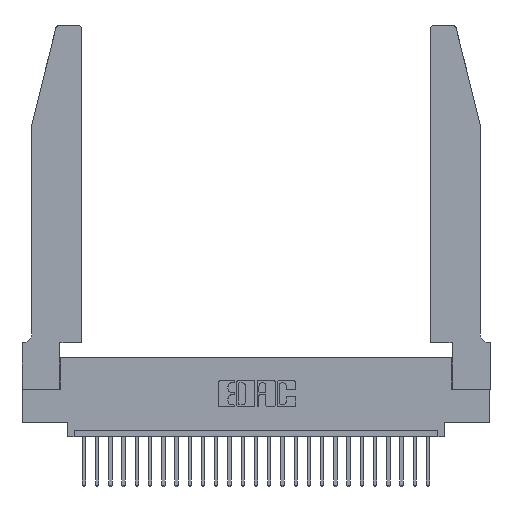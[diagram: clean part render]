
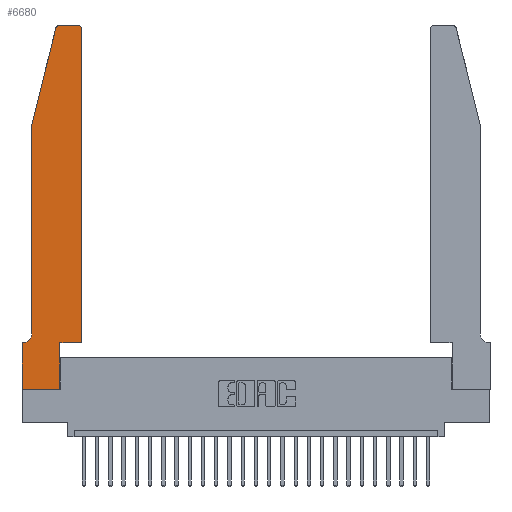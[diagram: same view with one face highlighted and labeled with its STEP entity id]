
A CAD part, top view. The second image highlights one B-rep face of the part: STEP entity #6680.
In plain terms, the highlighted planar face has unit normal (0, 0, 1).
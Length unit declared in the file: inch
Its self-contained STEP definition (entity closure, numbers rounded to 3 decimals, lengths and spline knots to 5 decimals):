
#149 = AXIS2_PLACEMENT_3D ( 'NONE', #14647, #1653, #1747 ) ;
#470 = ORIENTED_EDGE ( 'NONE', *, *, #9379, .T. ) ;
#734 = CIRCLE ( 'NONE', #1820, 0.03 ) ;
#816 = LINE ( 'NONE', #3206, #12697 ) ;
#826 = EDGE_CURVE ( 'NONE', #24561, #16037, #7368, .T. ) ;
#1127 = CARTESIAN_POINT ( 'NONE',  ( 0.2865, 0.35, 0.37 ) ) ;
#1187 = DIRECTION ( 'NONE',  ( 0., -1., 0. ) ) ;
#1245 = CIRCLE ( 'NONE', #149, 0.03 ) ;
#1454 = VERTEX_POINT ( 'NONE', #12712 ) ;
#1579 = CARTESIAN_POINT ( 'NONE',  ( 0.4505, 0.35, 0.37 ) ) ;
#1596 = CARTESIAN_POINT ( 'NONE',  ( 0., 0., 0.37 ) ) ;
#1653 = DIRECTION ( 'NONE',  ( 0., 0., 1. ) ) ;
#1747 = DIRECTION ( 'NONE',  ( 1., 0., 0. ) ) ;
#1820 = AXIS2_PLACEMENT_3D ( 'NONE', #4188, #27153, #19090 ) ;
#1962 = VECTOR ( 'NONE', #13848, 39.37008 ) ;
#3035 = DIRECTION ( 'NONE',  ( -1., 0., 0. ) ) ;
#3103 = EDGE_LOOP ( 'NONE', ( #20905, #11108, #470, #25592, #26043, #8160, #9879, #19861, #3679, #4403, #20275, #17504 ) ) ;
#3206 = CARTESIAN_POINT ( 'NONE',  ( 0.4505, 0.35, 0.37 ) ) ;
#3237 = VERTEX_POINT ( 'NONE', #6074 ) ;
#3348 = CARTESIAN_POINT ( 'NONE',  ( 0., 0., 0.37 ) ) ;
#3528 = VERTEX_POINT ( 'NONE', #17537 ) ;
#3679 = ORIENTED_EDGE ( 'NONE', *, *, #6394, .T. ) ;
#4188 = CARTESIAN_POINT ( 'NONE',  ( 0.4205, 2.72, 0.37 ) ) ;
#4379 = CARTESIAN_POINT ( 'NONE',  ( 0.4505, 2.72, 0.37 ) ) ;
#4403 = ORIENTED_EDGE ( 'NONE', *, *, #11843, .T. ) ;
#6074 = CARTESIAN_POINT ( 'NONE',  ( 0.25487, 2.72718, 0.37 ) ) ;
#6394 = EDGE_CURVE ( 'NONE', #25896, #17495, #16190, .T. ) ;
#6680 = ADVANCED_FACE ( 'NONE', ( #23380 ), #14019, .T. ) ;
#7368 = LINE ( 'NONE', #23674, #12301 ) ;
#8012 = CARTESIAN_POINT ( 'NONE',  ( 0., 0.35, 0.37 ) ) ;
#8160 = ORIENTED_EDGE ( 'NONE', *, *, #826, .T. ) ;
#8242 = CARTESIAN_POINT ( 'NONE',  ( 0.2605, 2.75, 0.37 ) ) ;
#8655 = CARTESIAN_POINT ( 'NONE',  ( 0.2865, 0.35, 0.37 ) ) ;
#8713 = LINE ( 'NONE', #3348, #20563 ) ;
#8955 = EDGE_CURVE ( 'NONE', #20782, #3528, #13169, .T. ) ;
#9379 = EDGE_CURVE ( 'NONE', #3237, #26907, #14814, .T. ) ;
#9433 = EDGE_CURVE ( 'NONE', #27029, #25896, #15794, .T. ) ;
#9781 = CARTESIAN_POINT ( 'NONE',  ( 0.0755, 2., 0.37 ) ) ;
#9879 = ORIENTED_EDGE ( 'NONE', *, *, #26983, .T. ) ;
#10260 = DIRECTION ( 'NONE',  ( 0., 1., 0. ) ) ;
#11108 = ORIENTED_EDGE ( 'NONE', *, *, #24088, .T. ) ;
#11843 = EDGE_CURVE ( 'NONE', #17495, #21492, #816, .T. ) ;
#12301 = VECTOR ( 'NONE', #25872, 39.37008 ) ;
#12697 = VECTOR ( 'NONE', #16104, 39.37008 ) ;
#12712 = CARTESIAN_POINT ( 'NONE',  ( 0.0755, 0.42, 0.37 ) ) ;
#12842 = AXIS2_PLACEMENT_3D ( 'NONE', #26087, #13269, #3035 ) ;
#13090 = EDGE_CURVE ( 'NONE', #24902, #20782, #734, .T. ) ;
#13169 = LINE ( 'NONE', #8242, #18742 ) ;
#13269 = DIRECTION ( 'NONE',  ( 0., 0., -1. ) ) ;
#13600 = EDGE_CURVE ( 'NONE', #21492, #24902, #19147, .T. ) ;
#13601 = CARTESIAN_POINT ( 'NONE',  ( 0.0755, 2., 0.37 ) ) ;
#13755 = CARTESIAN_POINT ( 'NONE',  ( 0., 0., 0.37 ) ) ;
#13848 = DIRECTION ( 'NONE',  ( 1., 0., 0. ) ) ;
#13943 = CIRCLE ( 'NONE', #12842, 0.07 ) ;
#13984 = CARTESIAN_POINT ( 'NONE',  ( 0.0055, 0.35, 0.37 ) ) ;
#14019 = PLANE ( 'NONE',  #22325 ) ;
#14143 = LINE ( 'NONE', #24428, #16114 ) ;
#14294 = DIRECTION ( 'NONE',  ( 0., 0., 1. ) ) ;
#14647 = CARTESIAN_POINT ( 'NONE',  ( 0.284, 2.72, 0.37 ) ) ;
#14814 = LINE ( 'NONE', #9781, #22678 ) ;
#15116 = CARTESIAN_POINT ( 'NONE',  ( 0.4205, 2.75, 0.37 ) ) ;
#15794 = LINE ( 'NONE', #13755, #1962 ) ;
#16037 = VERTEX_POINT ( 'NONE', #19517 ) ;
#16104 = DIRECTION ( 'NONE',  ( 1., 0., 0. ) ) ;
#16114 = VECTOR ( 'NONE', #1187, 39.37008 ) ;
#16190 = LINE ( 'NONE', #8655, #23710 ) ;
#16313 = DIRECTION ( 'NONE',  ( 1., 0., 0. ) ) ;
#16664 = CARTESIAN_POINT ( 'NONE',  ( 0.2865, 0., 0.37 ) ) ;
#16868 = DIRECTION ( 'NONE',  ( -1., 0., 0. ) ) ;
#17165 = VECTOR ( 'NONE', #10260, 39.37008 ) ;
#17495 = VERTEX_POINT ( 'NONE', #1127 ) ;
#17504 = ORIENTED_EDGE ( 'NONE', *, *, #13090, .T. ) ;
#17537 = CARTESIAN_POINT ( 'NONE',  ( 0.284, 2.75, 0.37 ) ) ;
#18742 = VECTOR ( 'NONE', #16868, 39.37008 ) ;
#18919 = EDGE_CURVE ( 'NONE', #1454, #24561, #13943, .T. ) ;
#19090 = DIRECTION ( 'NONE',  ( 1., 0., 0. ) ) ;
#19147 = LINE ( 'NONE', #1579, #17165 ) ;
#19517 = CARTESIAN_POINT ( 'NONE',  ( 0., 0.35, 0.37 ) ) ;
#19861 = ORIENTED_EDGE ( 'NONE', *, *, #9433, .T. ) ;
#20275 = ORIENTED_EDGE ( 'NONE', *, *, #13600, .T. ) ;
#20563 = VECTOR ( 'NONE', #22298, 39.37008 ) ;
#20782 = VERTEX_POINT ( 'NONE', #15116 ) ;
#20905 = ORIENTED_EDGE ( 'NONE', *, *, #8955, .T. ) ;
#21492 = VERTEX_POINT ( 'NONE', #24313 ) ;
#22298 = DIRECTION ( 'NONE',  ( 0., -1., 0. ) ) ;
#22325 = AXIS2_PLACEMENT_3D ( 'NONE', #8012, #14294, #16313 ) ;
#22678 = VECTOR ( 'NONE', #24445, 39.37008 ) ;
#23380 = FACE_OUTER_BOUND ( 'NONE', #3103, .T. ) ;
#23430 = DIRECTION ( 'NONE',  ( 0., 1., 0. ) ) ;
#23674 = CARTESIAN_POINT ( 'NONE',  ( 0.0755, 0.35, 0.37 ) ) ;
#23710 = VECTOR ( 'NONE', #23430, 39.37008 ) ;
#23928 = EDGE_CURVE ( 'NONE', #26907, #1454, #14143, .T. ) ;
#24088 = EDGE_CURVE ( 'NONE', #3528, #3237, #1245, .T. ) ;
#24313 = CARTESIAN_POINT ( 'NONE',  ( 0.4505, 0.35, 0.37 ) ) ;
#24428 = CARTESIAN_POINT ( 'NONE',  ( 0.0755, 2., 0.37 ) ) ;
#24445 = DIRECTION ( 'NONE',  ( -0.239, -0.971, 0. ) ) ;
#24561 = VERTEX_POINT ( 'NONE', #13984 ) ;
#24902 = VERTEX_POINT ( 'NONE', #4379 ) ;
#25592 = ORIENTED_EDGE ( 'NONE', *, *, #23928, .T. ) ;
#25872 = DIRECTION ( 'NONE',  ( -1., 0., 0. ) ) ;
#25896 = VERTEX_POINT ( 'NONE', #16664 ) ;
#26043 = ORIENTED_EDGE ( 'NONE', *, *, #18919, .T. ) ;
#26087 = CARTESIAN_POINT ( 'NONE',  ( 0.0055, 0.42, 0.37 ) ) ;
#26907 = VERTEX_POINT ( 'NONE', #13601 ) ;
#26983 = EDGE_CURVE ( 'NONE', #16037, #27029, #8713, .T. ) ;
#27029 = VERTEX_POINT ( 'NONE', #1596 ) ;
#27153 = DIRECTION ( 'NONE',  ( 0., 0., 1. ) ) ;
